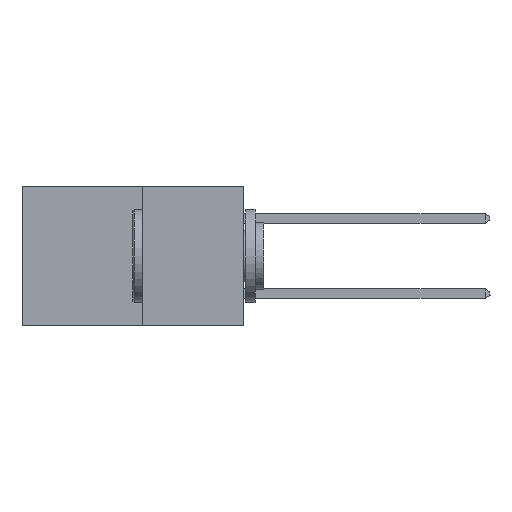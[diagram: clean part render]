
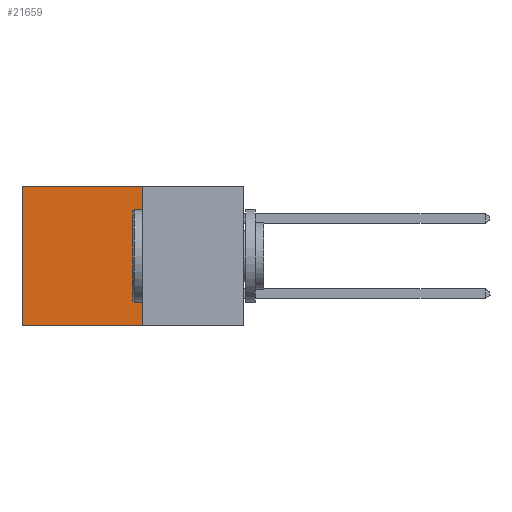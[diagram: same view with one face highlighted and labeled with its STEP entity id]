
A CAD part, left-side view. The second image highlights one B-rep face of the part: STEP entity #21659.
In plain terms, the highlighted planar face has unit normal (-1, 0, 0).
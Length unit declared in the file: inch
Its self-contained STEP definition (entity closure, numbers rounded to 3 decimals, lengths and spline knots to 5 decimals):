
#52 = VERTEX_POINT ( 'NONE', #15075 ) ;
#1265 = FACE_OUTER_BOUND ( 'NONE', #13185, .T. ) ;
#1570 = LINE ( 'NONE', #27482, #25282 ) ;
#1920 = VECTOR ( 'NONE', #25389, 39.37008 ) ;
#2678 = CARTESIAN_POINT ( 'NONE',  ( 0.277, 0.59, 0. ) ) ;
#3209 = AXIS2_PLACEMENT_3D ( 'NONE', #17662, #20280, #4551 ) ;
#4050 = CARTESIAN_POINT ( 'NONE',  ( 0.277, 0.27, -0.37 ) ) ;
#4522 = EDGE_CURVE ( 'NONE', #32264, #6860, #1570, .T. ) ;
#4551 = DIRECTION ( 'NONE',  ( 0., 0., -1. ) ) ;
#6860 = VERTEX_POINT ( 'NONE', #26767 ) ;
#7655 = CARTESIAN_POINT ( 'NONE',  ( 0.277, 0.27, 0. ) ) ;
#7788 = LINE ( 'NONE', #20818, #20912 ) ;
#12548 = EDGE_CURVE ( 'NONE', #52, #29561, #33704, .T. ) ;
#13143 = EDGE_CURVE ( 'NONE', #29561, #6860, #29646, .T. ) ;
#13185 = EDGE_LOOP ( 'NONE', ( #18077, #14381, #13258, #25517 ) ) ;
#13258 = ORIENTED_EDGE ( 'NONE', *, *, #29848, .F. ) ;
#14381 = ORIENTED_EDGE ( 'NONE', *, *, #4522, .F. ) ;
#15075 = CARTESIAN_POINT ( 'NONE',  ( 0.277, 0.27, 0. ) ) ;
#17662 = CARTESIAN_POINT ( 'NONE',  ( 0.277, 0.27, -0.37 ) ) ;
#18077 = ORIENTED_EDGE ( 'NONE', *, *, #13143, .T. ) ;
#20280 = DIRECTION ( 'NONE',  ( 1., 0., 0. ) ) ;
#20818 = CARTESIAN_POINT ( 'NONE',  ( 0.277, 0.27, -0.37 ) ) ;
#20912 = VECTOR ( 'NONE', #23386, 39.37008 ) ;
#21659 = ADVANCED_FACE ( 'NONE', ( #1265 ), #33095, .F. ) ;
#23291 = DIRECTION ( 'NONE',  ( 0., 1., 0. ) ) ;
#23386 = DIRECTION ( 'NONE',  ( 0., 0., -1. ) ) ;
#25282 = VECTOR ( 'NONE', #29665, 39.37008 ) ;
#25389 = DIRECTION ( 'NONE',  ( 0., 0., -1. ) ) ;
#25517 = ORIENTED_EDGE ( 'NONE', *, *, #12548, .T. ) ;
#26767 = CARTESIAN_POINT ( 'NONE',  ( 0.277, 0.59, -0.37 ) ) ;
#26837 = VECTOR ( 'NONE', #23291, 39.37008 ) ;
#27482 = CARTESIAN_POINT ( 'NONE',  ( 0.277, 0.27, -0.37 ) ) ;
#27971 = CARTESIAN_POINT ( 'NONE',  ( 0.277, 0.59, -0.37 ) ) ;
#29561 = VERTEX_POINT ( 'NONE', #2678 ) ;
#29646 = LINE ( 'NONE', #27971, #1920 ) ;
#29665 = DIRECTION ( 'NONE',  ( 0., 1., 0. ) ) ;
#29848 = EDGE_CURVE ( 'NONE', #52, #32264, #7788, .T. ) ;
#32264 = VERTEX_POINT ( 'NONE', #4050 ) ;
#33095 = PLANE ( 'NONE',  #3209 ) ;
#33704 = LINE ( 'NONE', #7655, #26837 ) ;
